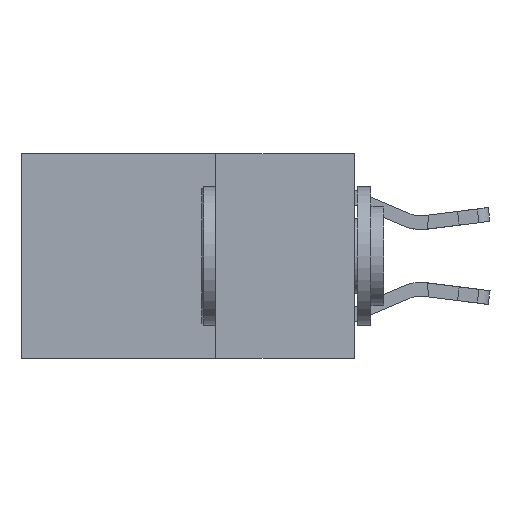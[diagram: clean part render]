
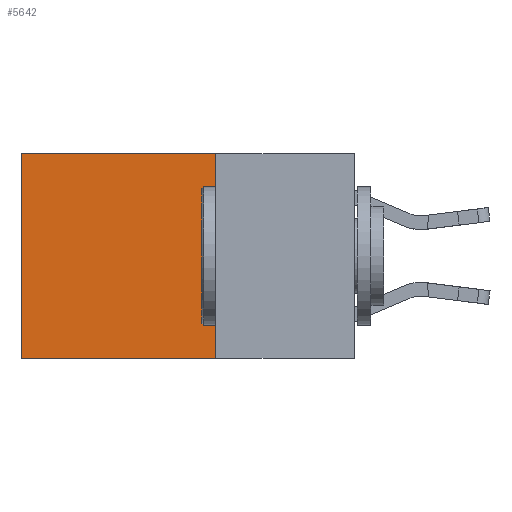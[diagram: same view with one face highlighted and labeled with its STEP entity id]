
A CAD part, left-side view. The second image highlights one B-rep face of the part: STEP entity #5642.
In plain terms, the highlighted planar face has unit normal (-1, 0, 0).
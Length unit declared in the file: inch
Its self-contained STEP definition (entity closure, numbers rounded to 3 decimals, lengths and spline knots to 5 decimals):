
#1560 = VECTOR ( 'NONE', #6276, 39.37008 ) ;
#2377 = EDGE_CURVE ( 'NONE', #14990, #18979, #2445, .T. ) ;
#2445 = LINE ( 'NONE', #11578, #1560 ) ;
#3355 = PLANE ( 'NONE',  #18611 ) ;
#3533 = CARTESIAN_POINT ( 'NONE',  ( 0.2625, 0.25, 0. ) ) ;
#4644 = CARTESIAN_POINT ( 'NONE',  ( 0.2625, 0.25, -0.37 ) ) ;
#4772 = EDGE_CURVE ( 'NONE', #15286, #14990, #22269, .T. ) ;
#5442 = DIRECTION ( 'NONE',  ( 0., 1., 0. ) ) ;
#5642 = ADVANCED_FACE ( 'NONE', ( #16079 ), #3355, .F. ) ;
#5690 = VECTOR ( 'NONE', #8196, 39.37008 ) ;
#6276 = DIRECTION ( 'NONE',  ( 0., 0., -1. ) ) ;
#7418 = DIRECTION ( 'NONE',  ( 0., 0., -1. ) ) ;
#8196 = DIRECTION ( 'NONE',  ( 0., 1., 0. ) ) ;
#9592 = CARTESIAN_POINT ( 'NONE',  ( 0.2625, 0.6, -0.37 ) ) ;
#10187 = EDGE_CURVE ( 'NONE', #22807, #18979, #15924, .T. ) ;
#10569 = ORIENTED_EDGE ( 'NONE', *, *, #10187, .F. ) ;
#10909 = EDGE_LOOP ( 'NONE', ( #16061, #10569, #21305, #21767 ) ) ;
#11578 = CARTESIAN_POINT ( 'NONE',  ( 0.2625, 0.6, 0. ) ) ;
#13400 = LINE ( 'NONE', #23525, #23596 ) ;
#14333 = DIRECTION ( 'NONE',  ( 0., 0., -1. ) ) ;
#14779 = CARTESIAN_POINT ( 'NONE',  ( 0.2625, 0.25, 0. ) ) ;
#14990 = VERTEX_POINT ( 'NONE', #15382 ) ;
#15286 = VERTEX_POINT ( 'NONE', #17165 ) ;
#15382 = CARTESIAN_POINT ( 'NONE',  ( 0.2625, 0.6, 0. ) ) ;
#15924 = LINE ( 'NONE', #4644, #5690 ) ;
#16061 = ORIENTED_EDGE ( 'NONE', *, *, #2377, .T. ) ;
#16079 = FACE_OUTER_BOUND ( 'NONE', #10909, .T. ) ;
#17165 = CARTESIAN_POINT ( 'NONE',  ( 0.2625, 0.25, 0. ) ) ;
#18329 = DIRECTION ( 'NONE',  ( 1., 0., 0. ) ) ;
#18611 = AXIS2_PLACEMENT_3D ( 'NONE', #3533, #18329, #7418 ) ;
#18979 = VERTEX_POINT ( 'NONE', #9592 ) ;
#21120 = VECTOR ( 'NONE', #5442, 39.37008 ) ;
#21305 = ORIENTED_EDGE ( 'NONE', *, *, #24160, .F. ) ;
#21534 = CARTESIAN_POINT ( 'NONE',  ( 0.2625, 0.25, -0.37 ) ) ;
#21767 = ORIENTED_EDGE ( 'NONE', *, *, #4772, .T. ) ;
#22269 = LINE ( 'NONE', #14779, #21120 ) ;
#22807 = VERTEX_POINT ( 'NONE', #21534 ) ;
#23525 = CARTESIAN_POINT ( 'NONE',  ( 0.2625, 0.25, 0. ) ) ;
#23596 = VECTOR ( 'NONE', #14333, 39.37008 ) ;
#24160 = EDGE_CURVE ( 'NONE', #15286, #22807, #13400, .T. ) ;
